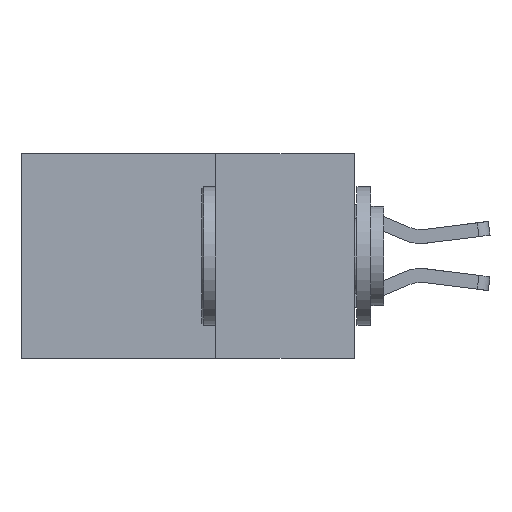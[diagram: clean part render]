
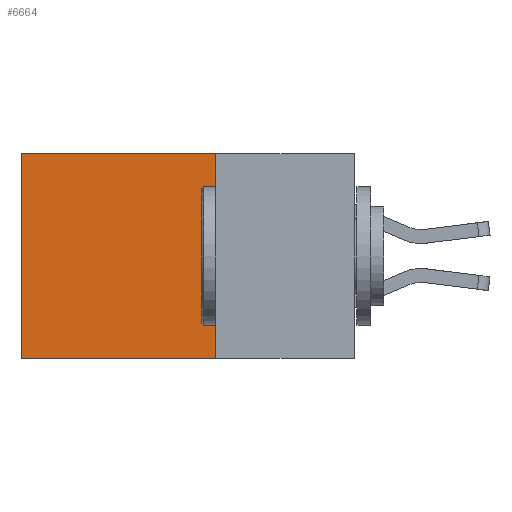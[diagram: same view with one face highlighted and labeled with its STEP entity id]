
A CAD part, left-side view. The second image highlights one B-rep face of the part: STEP entity #6664.
In plain terms, the highlighted planar face has unit normal (-1, 0, 0).
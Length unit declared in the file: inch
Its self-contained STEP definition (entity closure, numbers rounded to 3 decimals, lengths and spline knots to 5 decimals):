
#657 = DIRECTION ( 'NONE',  ( 0., 1., 0. ) ) ;
#715 = CARTESIAN_POINT ( 'NONE',  ( 0.2615, 0.25, -0.37 ) ) ;
#721 = CARTESIAN_POINT ( 'NONE',  ( 0.2615, 0.25, 0. ) ) ;
#990 = EDGE_CURVE ( 'NONE', #1274, #2847, #3779, .T. ) ;
#1130 = LINE ( 'NONE', #8218, #4114 ) ;
#1274 = VERTEX_POINT ( 'NONE', #721 ) ;
#1325 = EDGE_CURVE ( 'NONE', #2847, #6938, #6150, .T. ) ;
#1421 = DIRECTION ( 'NONE',  ( 0., 1., 0. ) ) ;
#1509 = VECTOR ( 'NONE', #657, 39.37008 ) ;
#1885 = DIRECTION ( 'NONE',  ( 0., 0., -1. ) ) ;
#2071 = CARTESIAN_POINT ( 'NONE',  ( 0.2615, 0.6, -0.37 ) ) ;
#2847 = VERTEX_POINT ( 'NONE', #7346 ) ;
#3460 = AXIS2_PLACEMENT_3D ( 'NONE', #7103, #6345, #7745 ) ;
#3471 = EDGE_CURVE ( 'NONE', #5735, #6938, #3599, .T. ) ;
#3599 = LINE ( 'NONE', #715, #1509 ) ;
#3779 = LINE ( 'NONE', #7716, #5235 ) ;
#3969 = FACE_OUTER_BOUND ( 'NONE', #6879, .T. ) ;
#4114 = VECTOR ( 'NONE', #1885, 39.37008 ) ;
#4222 = EDGE_CURVE ( 'NONE', #1274, #5735, #1130, .T. ) ;
#5054 = ORIENTED_EDGE ( 'NONE', *, *, #3471, .F. ) ;
#5235 = VECTOR ( 'NONE', #1421, 39.37008 ) ;
#5258 = DIRECTION ( 'NONE',  ( 0., 0., -1. ) ) ;
#5600 = ORIENTED_EDGE ( 'NONE', *, *, #1325, .T. ) ;
#5617 = ORIENTED_EDGE ( 'NONE', *, *, #990, .T. ) ;
#5673 = PLANE ( 'NONE',  #3460 ) ;
#5735 = VERTEX_POINT ( 'NONE', #6931 ) ;
#6150 = LINE ( 'NONE', #2071, #9230 ) ;
#6345 = DIRECTION ( 'NONE',  ( 1., 0., 0. ) ) ;
#6664 = ADVANCED_FACE ( 'NONE', ( #3969 ), #5673, .F. ) ;
#6879 = EDGE_LOOP ( 'NONE', ( #5600, #5054, #8870, #5617 ) ) ;
#6931 = CARTESIAN_POINT ( 'NONE',  ( 0.2615, 0.25, -0.37 ) ) ;
#6932 = CARTESIAN_POINT ( 'NONE',  ( 0.2615, 0.6, -0.37 ) ) ;
#6938 = VERTEX_POINT ( 'NONE', #6932 ) ;
#7103 = CARTESIAN_POINT ( 'NONE',  ( 0.2615, 0.25, -0.37 ) ) ;
#7346 = CARTESIAN_POINT ( 'NONE',  ( 0.2615, 0.6, 0. ) ) ;
#7716 = CARTESIAN_POINT ( 'NONE',  ( 0.2615, 0.25, 0. ) ) ;
#7745 = DIRECTION ( 'NONE',  ( 0., 0., -1. ) ) ;
#8218 = CARTESIAN_POINT ( 'NONE',  ( 0.2615, 0.25, -0.37 ) ) ;
#8870 = ORIENTED_EDGE ( 'NONE', *, *, #4222, .F. ) ;
#9230 = VECTOR ( 'NONE', #5258, 39.37008 ) ;
